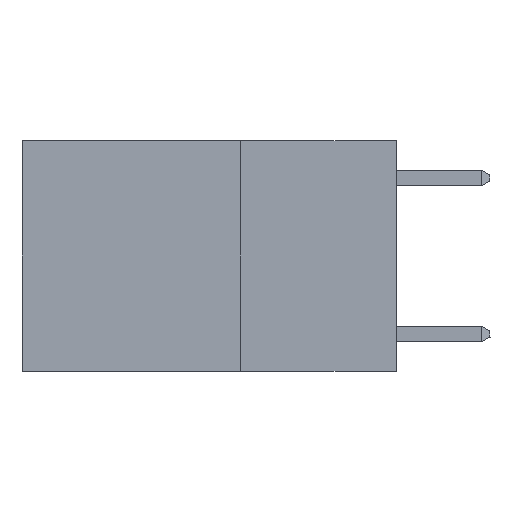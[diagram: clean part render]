
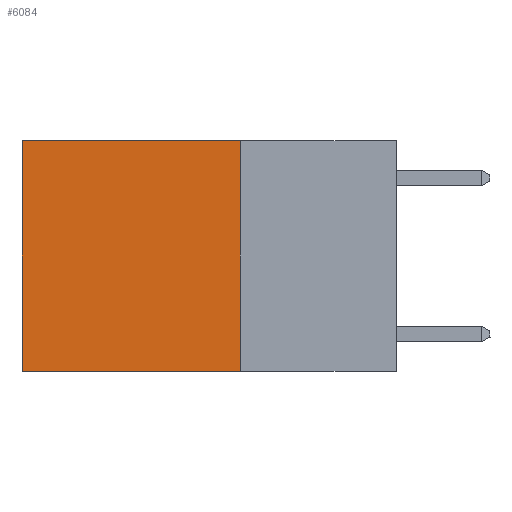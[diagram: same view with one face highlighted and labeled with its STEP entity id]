
A CAD part, left-side view. The second image highlights one B-rep face of the part: STEP entity #6084.
In plain terms, the highlighted planar face has unit normal (-1, 0, 0).
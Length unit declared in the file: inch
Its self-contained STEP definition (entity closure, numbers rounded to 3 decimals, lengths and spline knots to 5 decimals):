
#105 = CARTESIAN_POINT ( 'NONE',  ( 0.2625, 0.6, 0. ) ) ;
#577 = ORIENTED_EDGE ( 'NONE', *, *, #2972, .T. ) ;
#963 = ORIENTED_EDGE ( 'NONE', *, *, #9503, .F. ) ;
#994 = DIRECTION ( 'NONE',  ( 0., 1., 0. ) ) ;
#1782 = VECTOR ( 'NONE', #6020, 39.37008 ) ;
#1850 = PLANE ( 'NONE',  #7271 ) ;
#2732 = CARTESIAN_POINT ( 'NONE',  ( 0.2625, 0.6, 0. ) ) ;
#2799 = CARTESIAN_POINT ( 'NONE',  ( 0.2625, 0.25, 0. ) ) ;
#2972 = EDGE_CURVE ( 'NONE', #4128, #5931, #3517, .T. ) ;
#3382 = DIRECTION ( 'NONE',  ( 0., 0., -1. ) ) ;
#3517 = LINE ( 'NONE', #4270, #6650 ) ;
#3522 = VERTEX_POINT ( 'NONE', #5169 ) ;
#4021 = LINE ( 'NONE', #7574, #9473 ) ;
#4128 = VERTEX_POINT ( 'NONE', #2799 ) ;
#4270 = CARTESIAN_POINT ( 'NONE',  ( 0.2625, 0.25, 0. ) ) ;
#4835 = EDGE_CURVE ( 'NONE', #6556, #3522, #7100, .T. ) ;
#5169 = CARTESIAN_POINT ( 'NONE',  ( 0.2625, 0.6, -0.37 ) ) ;
#5931 = VERTEX_POINT ( 'NONE', #2732 ) ;
#5955 = CARTESIAN_POINT ( 'NONE',  ( 0.2625, 0.25, -0.37 ) ) ;
#6020 = DIRECTION ( 'NONE',  ( 0., 1., 0. ) ) ;
#6084 = ADVANCED_FACE ( 'NONE', ( #8951 ), #1850, .F. ) ;
#6147 = DIRECTION ( 'NONE',  ( 1., 0., 0. ) ) ;
#6556 = VERTEX_POINT ( 'NONE', #5955 ) ;
#6650 = VECTOR ( 'NONE', #994, 39.37008 ) ;
#6719 = ORIENTED_EDGE ( 'NONE', *, *, #4835, .F. ) ;
#6791 = VECTOR ( 'NONE', #3382, 39.37008 ) ;
#7100 = LINE ( 'NONE', #9115, #1782 ) ;
#7117 = LINE ( 'NONE', #105, #6791 ) ;
#7271 = AXIS2_PLACEMENT_3D ( 'NONE', #11159, #6147, #13225 ) ;
#7574 = CARTESIAN_POINT ( 'NONE',  ( 0.2625, 0.25, 0. ) ) ;
#8539 = DIRECTION ( 'NONE',  ( 0., 0., -1. ) ) ;
#8951 = FACE_OUTER_BOUND ( 'NONE', #12493, .T. ) ;
#9115 = CARTESIAN_POINT ( 'NONE',  ( 0.2625, 0.25, -0.37 ) ) ;
#9473 = VECTOR ( 'NONE', #8539, 39.37008 ) ;
#9503 = EDGE_CURVE ( 'NONE', #4128, #6556, #4021, .T. ) ;
#11159 = CARTESIAN_POINT ( 'NONE',  ( 0.2625, 0.25, 0. ) ) ;
#11572 = ORIENTED_EDGE ( 'NONE', *, *, #13042, .T. ) ;
#12493 = EDGE_LOOP ( 'NONE', ( #11572, #6719, #963, #577 ) ) ;
#13042 = EDGE_CURVE ( 'NONE', #5931, #3522, #7117, .T. ) ;
#13225 = DIRECTION ( 'NONE',  ( 0., 0., -1. ) ) ;
